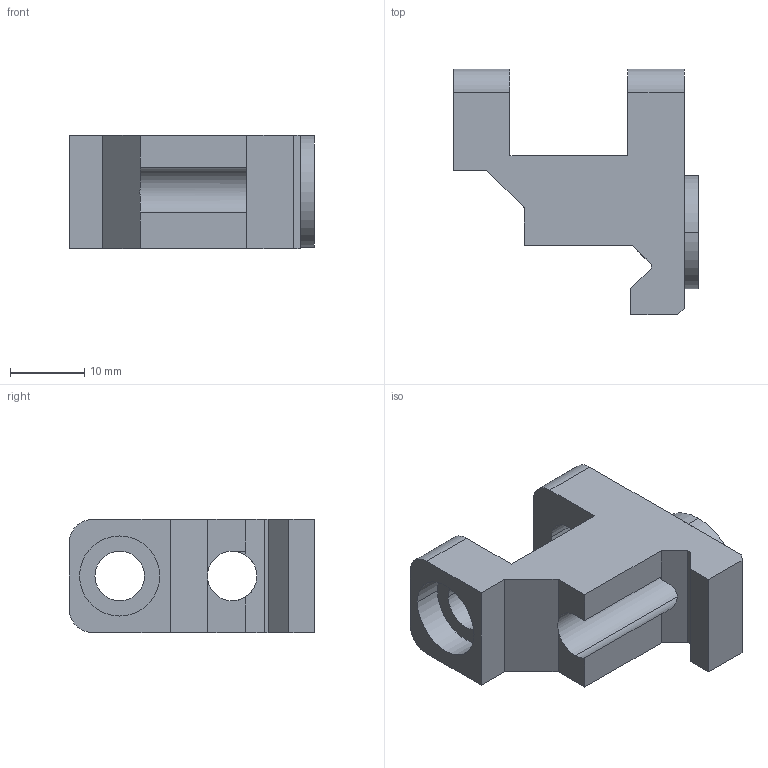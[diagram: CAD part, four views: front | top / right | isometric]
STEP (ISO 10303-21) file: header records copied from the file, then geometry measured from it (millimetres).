
FILE_DESCRIPTION (( 'STEP AP203' ), '1' );
FILE_NAME ('AF-WF-GS-PRT-006-STEP.STEP', '2020-07-21T22:58:59', ( '' ), ( '' ), 'SwSTEP 2.0', 'SolidWorks 2018', '' );
FILE_SCHEMA (( 'CONFIG_CONTROL_DESIGN' ));
Length unit declared in the file: inch
Products named in the file (1): AF-WF-GS-PRT-006-STEP
Bounding box: 32.96 x 33.07 x 15.24 mm (x, y, z)
Volume: 5851.8 mm3; surface area: 4106.8 mm2
Topology: 1 solids, 1 shells, 54 faces, 146 edges, 96 vertices
Faces by surface type: plane 38, cylinder 16
Entity records: 1783 total; most frequent: CARTESIAN_POINT 303, ORIENTED_EDGE 292, DIRECTION 288, EDGE_CURVE 146, VECTOR 110, LINE 110, VERTEX_POINT 96, AXIS2_PLACEMENT_3D 89
